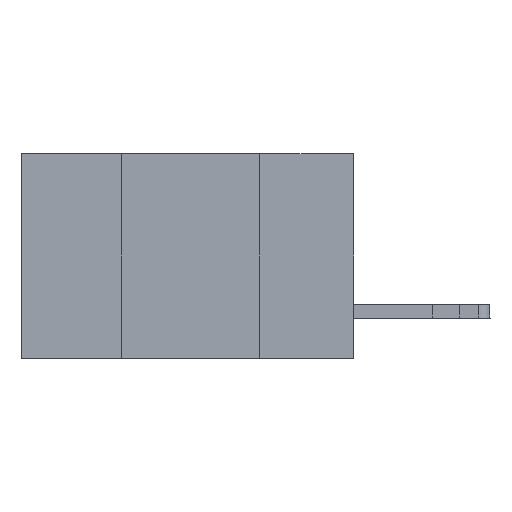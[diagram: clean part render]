
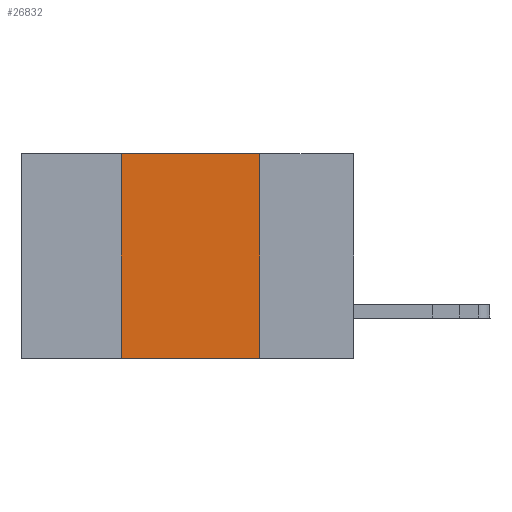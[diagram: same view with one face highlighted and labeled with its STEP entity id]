
A CAD part, left-side view. The second image highlights one B-rep face of the part: STEP entity #26832.
In plain terms, the highlighted planar face has unit normal (-1, 0, 0).
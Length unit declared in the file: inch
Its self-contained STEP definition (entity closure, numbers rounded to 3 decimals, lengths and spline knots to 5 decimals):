
#28 = CARTESIAN_POINT ( 'NONE',  ( 0., 0.6, -0.37 ) ) ;
#446 = EDGE_CURVE ( 'NONE', #25263, #26129, #10812, .T. ) ;
#2048 = DIRECTION ( 'NONE',  ( 0., 0., 1. ) ) ;
#2528 = VERTEX_POINT ( 'NONE', #29782 ) ;
#4762 = VERTEX_POINT ( 'NONE', #12550 ) ;
#5967 = FACE_OUTER_BOUND ( 'NONE', #19369, .T. ) ;
#7648 = CARTESIAN_POINT ( 'NONE',  ( 0., 0.42, 0. ) ) ;
#8116 = VECTOR ( 'NONE', #23699, 39.37008 ) ;
#8546 = VECTOR ( 'NONE', #14265, 39.37008 ) ;
#10177 = DIRECTION ( 'NONE',  ( 0., -1., 0. ) ) ;
#10303 = VECTOR ( 'NONE', #10177, 39.37008 ) ;
#10812 = LINE ( 'NONE', #20903, #8116 ) ;
#10839 = VECTOR ( 'NONE', #2048, 39.37008 ) ;
#11057 = CARTESIAN_POINT ( 'NONE',  ( 0., 0.17, 0. ) ) ;
#12338 = DIRECTION ( 'NONE',  ( 0., 0., -1. ) ) ;
#12550 = CARTESIAN_POINT ( 'NONE',  ( 0., 0.42, -0.37 ) ) ;
#14265 = DIRECTION ( 'NONE',  ( 0., -1., 0. ) ) ;
#17321 = ORIENTED_EDGE ( 'NONE', *, *, #30255, .T. ) ;
#17862 = LINE ( 'NONE', #29867, #10303 ) ;
#19369 = EDGE_LOOP ( 'NONE', ( #30762, #32380, #19831, #17321 ) ) ;
#19831 = ORIENTED_EDGE ( 'NONE', *, *, #29562, .F. ) ;
#20170 = LINE ( 'NONE', #7648, #10839 ) ;
#20747 = CARTESIAN_POINT ( 'NONE',  ( 0., 0.6, 0. ) ) ;
#20903 = CARTESIAN_POINT ( 'NONE',  ( 0., 0.17, 0. ) ) ;
#23593 = LINE ( 'NONE', #28, #8546 ) ;
#23699 = DIRECTION ( 'NONE',  ( 0., 0., -1. ) ) ;
#25263 = VERTEX_POINT ( 'NONE', #11057 ) ;
#25740 = AXIS2_PLACEMENT_3D ( 'NONE', #20747, #29166, #12338 ) ;
#26129 = VERTEX_POINT ( 'NONE', #34232 ) ;
#26368 = PLANE ( 'NONE',  #25740 ) ;
#26832 = ADVANCED_FACE ( 'NONE', ( #5967 ), #26368, .F. ) ;
#29166 = DIRECTION ( 'NONE',  ( 1., 0., 0. ) ) ;
#29562 = EDGE_CURVE ( 'NONE', #4762, #2528, #20170, .T. ) ;
#29782 = CARTESIAN_POINT ( 'NONE',  ( 0., 0.42, 0. ) ) ;
#29867 = CARTESIAN_POINT ( 'NONE',  ( 0., 0.6, 0. ) ) ;
#30255 = EDGE_CURVE ( 'NONE', #4762, #26129, #23593, .T. ) ;
#30762 = ORIENTED_EDGE ( 'NONE', *, *, #446, .F. ) ;
#31321 = EDGE_CURVE ( 'NONE', #2528, #25263, #17862, .T. ) ;
#32380 = ORIENTED_EDGE ( 'NONE', *, *, #31321, .F. ) ;
#34232 = CARTESIAN_POINT ( 'NONE',  ( 0., 0.17, -0.37 ) ) ;
